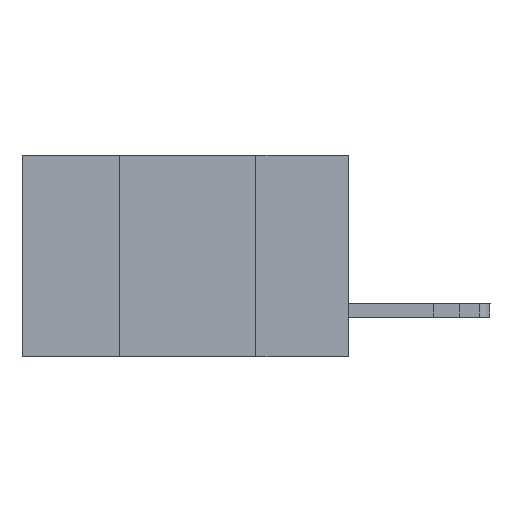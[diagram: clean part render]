
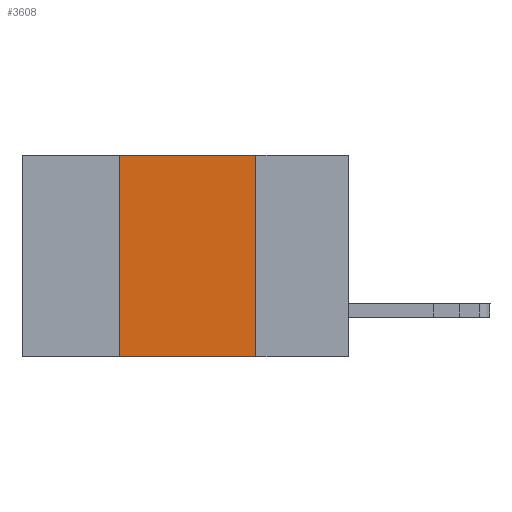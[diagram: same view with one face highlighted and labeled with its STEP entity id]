
A CAD part, left-side view. The second image highlights one B-rep face of the part: STEP entity #3608.
In plain terms, the highlighted planar face has unit normal (-1, 0, 0).
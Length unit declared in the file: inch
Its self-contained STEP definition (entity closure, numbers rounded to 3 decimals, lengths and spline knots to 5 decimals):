
#1149 = FACE_OUTER_BOUND ( 'NONE', #4557, .T. ) ;
#1216 = DIRECTION ( 'NONE',  ( 1., 0., 0. ) ) ;
#1275 = DIRECTION ( 'NONE',  ( 0., 0., 1. ) ) ;
#1381 = EDGE_CURVE ( 'NONE', #12510, #11610, #2030, .T. ) ;
#1407 = VECTOR ( 'NONE', #3097, 39.37008 ) ;
#2030 = LINE ( 'NONE', #4390, #1407 ) ;
#2434 = LINE ( 'NONE', #8985, #7309 ) ;
#3097 = DIRECTION ( 'NONE',  ( 0., -1., 0. ) ) ;
#3342 = AXIS2_PLACEMENT_3D ( 'NONE', #11964, #1216, #4367 ) ;
#3427 = VERTEX_POINT ( 'NONE', #13612 ) ;
#3608 = ADVANCED_FACE ( 'NONE', ( #1149 ), #8831, .F. ) ;
#4367 = DIRECTION ( 'NONE',  ( 0., 0., -1. ) ) ;
#4390 = CARTESIAN_POINT ( 'NONE',  ( 0., 0.6, -0.37 ) ) ;
#4557 = EDGE_LOOP ( 'NONE', ( #11893, #8470, #5301, #11733 ) ) ;
#4815 = VECTOR ( 'NONE', #9112, 39.37008 ) ;
#5301 = ORIENTED_EDGE ( 'NONE', *, *, #11650, .F. ) ;
#6817 = VERTEX_POINT ( 'NONE', #7842 ) ;
#7309 = VECTOR ( 'NONE', #13320, 39.37008 ) ;
#7761 = CARTESIAN_POINT ( 'NONE',  ( 0., 0.17, -0.37 ) ) ;
#7842 = CARTESIAN_POINT ( 'NONE',  ( 0., 0.42, 0. ) ) ;
#8470 = ORIENTED_EDGE ( 'NONE', *, *, #11679, .F. ) ;
#8831 = PLANE ( 'NONE',  #3342 ) ;
#8985 = CARTESIAN_POINT ( 'NONE',  ( 0., 0.17, 0. ) ) ;
#9112 = DIRECTION ( 'NONE',  ( 0., -1., 0. ) ) ;
#9182 = CARTESIAN_POINT ( 'NONE',  ( 0., 0.6, 0. ) ) ;
#10398 = LINE ( 'NONE', #9182, #4815 ) ;
#10968 = CARTESIAN_POINT ( 'NONE',  ( 0., 0.42, 0. ) ) ;
#11185 = EDGE_CURVE ( 'NONE', #3427, #11610, #2434, .T. ) ;
#11242 = LINE ( 'NONE', #10968, #13656 ) ;
#11610 = VERTEX_POINT ( 'NONE', #7761 ) ;
#11650 = EDGE_CURVE ( 'NONE', #12510, #6817, #11242, .T. ) ;
#11679 = EDGE_CURVE ( 'NONE', #6817, #3427, #10398, .T. ) ;
#11733 = ORIENTED_EDGE ( 'NONE', *, *, #1381, .T. ) ;
#11893 = ORIENTED_EDGE ( 'NONE', *, *, #11185, .F. ) ;
#11964 = CARTESIAN_POINT ( 'NONE',  ( 0., 0.6, 0. ) ) ;
#12497 = CARTESIAN_POINT ( 'NONE',  ( 0., 0.42, -0.37 ) ) ;
#12510 = VERTEX_POINT ( 'NONE', #12497 ) ;
#13320 = DIRECTION ( 'NONE',  ( 0., 0., -1. ) ) ;
#13612 = CARTESIAN_POINT ( 'NONE',  ( 0., 0.17, 0. ) ) ;
#13656 = VECTOR ( 'NONE', #1275, 39.37008 ) ;
